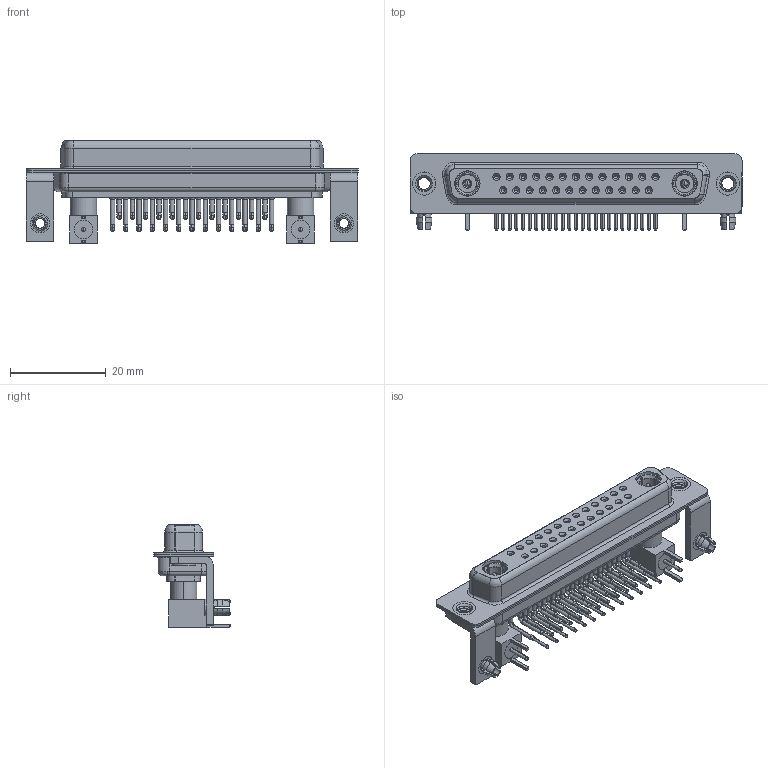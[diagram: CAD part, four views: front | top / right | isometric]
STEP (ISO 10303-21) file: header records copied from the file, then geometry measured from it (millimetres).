
FILE_DESCRIPTION (( 'STEP AP203' ), '1' );
FILE_NAME ('630-27W2640-7NB.STEP', '2022-06-07T18:23:45', ( '' ), ( '' ), 'SwSTEP 2.0', 'SolidWorks 2020', '' );
FILE_SCHEMA (( 'CONFIG_CONTROL_DESIGN' ));
Length unit declared in the file: millimetre
Products named in the file (17): RA Back Shell; Co-Ax Plug Assy_RA; Insulator Pin_Straight PC Tail; Locking Collar; 630Combo Threaded Rivet_B; 630Combo Shell Front_37 Contacts; 630-27W2640-7NB; Co-Ax Plug_RA PC Tail; 630Combo Contact Row 1; Pin_RA; Insulator RA Pin; 630Combo Contact Row 2; 630Combo Board Lock; 630Combo Housing_27W2; 630Combo Shell Rear_37 Contacts; 630Combo Stabilizer Bracket
Assembly tree (48 placements, depth 3):
  630-27W2640-7NB
    630Combo Housing_27W2
    630Combo Shell Front_37 Contacts
    630Combo Shell Rear_37 Contacts
    630Combo Threaded Rivet_B  x2
    630Combo Stabilizer Bracket  x2
    630Combo Board Lock  x2
    Co-Ax Plug Assy_RA
      Co-Ax Plug_RA PC Tail
      Insulator Pin_Straight PC Tail
      Pin_RA
      Locking Collar
      RA Back Shell
      Insulator RA Pin
    Co-Ax Plug Assy_RA
      Co-Ax Plug_RA PC Tail
      Insulator Pin_Straight PC Tail
      Pin_RA
      Locking Collar
      RA Back Shell
      Insulator RA Pin
    630Combo Contact Row 1  x13
    630Combo Contact Row 2  x12
Bounding box: 69.4 x 16 x 21.41 mm (x, y, z)
Volume: 6304.3 mm3; surface area: 14592.6 mm2
Topology: 46 solids, 46 shells, 2070 faces, 5206 edges, 3280 vertices
Faces by surface type: cylinder 892, plane 644, cone 349, bspline 108, torus 69, sphere 8
Entity records: 30507 total; most frequent: CARTESIAN_POINT 6413, DIRECTION 4921, ORIENTED_EDGE 4166, EDGE_CURVE 2083, AXIS2_PLACEMENT_3D 2027, VERTEX_POINT 1329, CIRCLE 1097, EDGE_LOOP 1078
